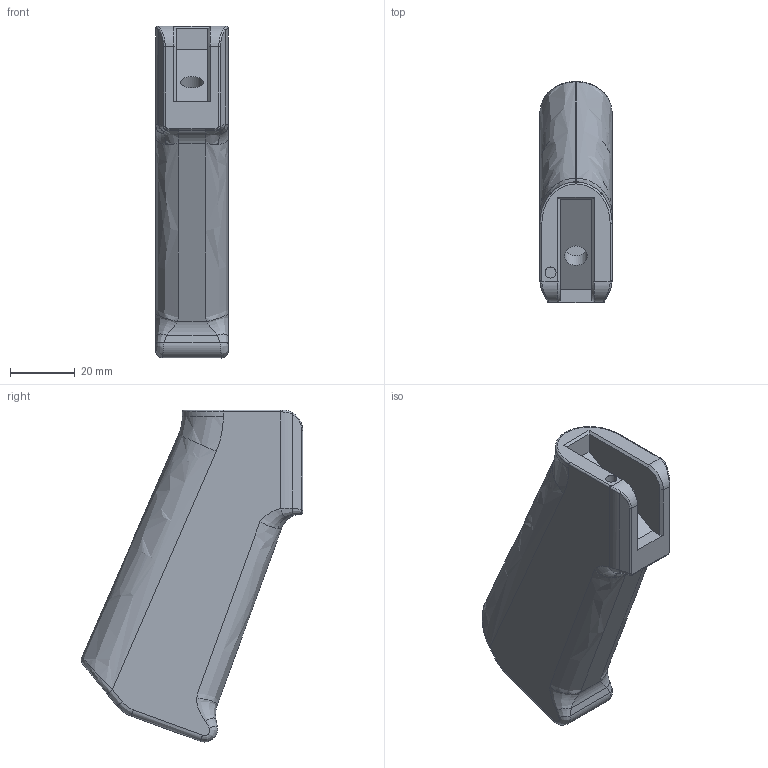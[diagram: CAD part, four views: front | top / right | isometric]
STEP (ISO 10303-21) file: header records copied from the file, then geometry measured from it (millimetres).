
FILE_DESCRIPTION(/* description */ (''),/* implementation_level */ '2;1');
FILE_NAME(/* name */ 'Standard Grip.step',/* time_stamp */ '2021-02-28T22:56:19-05:00',/* author */ (''),/* organization */ (''),/* preprocessor_version */ 'ST-DEVELOPER v18.1',/* originating_system */ 'Autodesk Translation Framework v9.7.1.1290',/* authorisation */ '');
FILE_SCHEMA (('AUTOMOTIVE_DESIGN { 1 0 10303 214 3 1 1 }'));
Length unit declared in the file: millimetre
Products named in the file (1): Standard Grip
Bounding box: 22.33 x 68.42 x 102.58 mm (x, y, z)
Volume: 54809.7 mm3; surface area: 20192.4 mm2
Topology: 1 solids, 1 shells, 277 faces, 717 edges, 451 vertices
Faces by surface type: bspline 116, plane 114, cylinder 40, torus 4, cone 3
Full cylindrical faces by diameter (mm): 3.4 x1, 7 x1
Entity records: 11434 total; most frequent: CARTESIAN_POINT 5413, ORIENTED_EDGE 1434, DIRECTION 894, EDGE_CURVE 717, VERTEX_POINT 451, LINE 394, VECTOR 394, EDGE_LOOP 288
